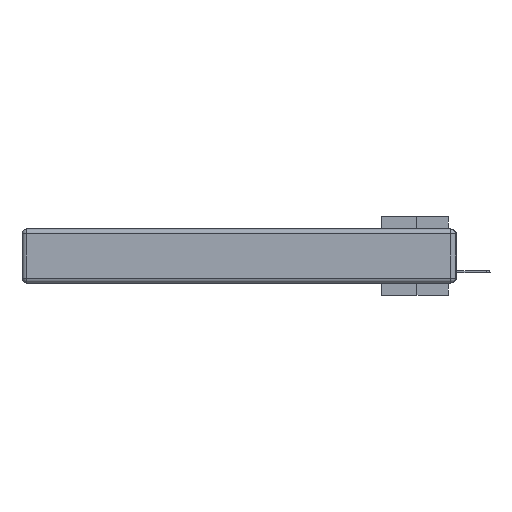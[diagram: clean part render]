
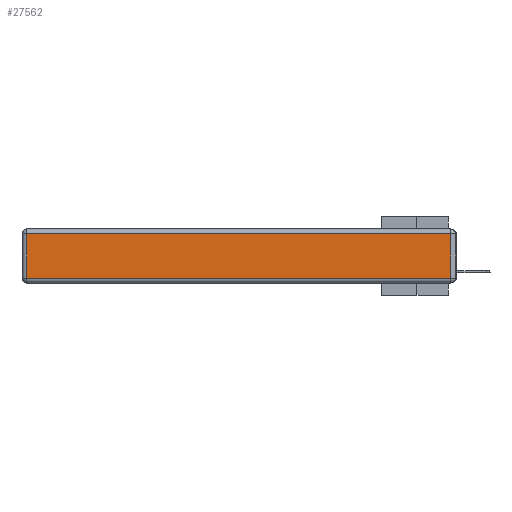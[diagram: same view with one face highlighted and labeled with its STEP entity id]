
A CAD part, left-side view. The second image highlights one B-rep face of the part: STEP entity #27562.
In plain terms, the highlighted planar face has unit normal (-1, 0, 0).
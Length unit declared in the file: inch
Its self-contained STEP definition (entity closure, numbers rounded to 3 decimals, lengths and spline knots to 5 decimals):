
#296 = EDGE_CURVE ( 'NONE', #33490, #36458, #23448, .T. ) ;
#3429 = DIRECTION ( 'NONE',  ( 0., -1., 0. ) ) ;
#3617 = AXIS2_PLACEMENT_3D ( 'NONE', #33273, #27860, #33509 ) ;
#4100 = LINE ( 'NONE', #26617, #32012 ) ;
#4236 = CARTESIAN_POINT ( 'NONE',  ( 0., 0.03, -0.03 ) ) ;
#4678 = EDGE_LOOP ( 'NONE', ( #19805, #11359, #30119, #31529 ) ) ;
#9135 = CARTESIAN_POINT ( 'NONE',  ( 0., 2.72, -0.313 ) ) ;
#11359 = ORIENTED_EDGE ( 'NONE', *, *, #21497, .T. ) ;
#11475 = DIRECTION ( 'NONE',  ( 0., 1., 0. ) ) ;
#11757 = EDGE_CURVE ( 'NONE', #20906, #33490, #23233, .T. ) ;
#13378 = FACE_OUTER_BOUND ( 'NONE', #4678, .T. ) ;
#16796 = CARTESIAN_POINT ( 'NONE',  ( 0., 0.03, -0.343 ) ) ;
#18258 = VECTOR ( 'NONE', #11475, 39.37008 ) ;
#18913 = VERTEX_POINT ( 'NONE', #28875 ) ;
#19805 = ORIENTED_EDGE ( 'NONE', *, *, #25335, .T. ) ;
#20906 = VERTEX_POINT ( 'NONE', #4236 ) ;
#21497 = EDGE_CURVE ( 'NONE', #18913, #20906, #30073, .T. ) ;
#22880 = CARTESIAN_POINT ( 'NONE',  ( 0., 2.72, -0.03 ) ) ;
#23233 = LINE ( 'NONE', #36907, #18258 ) ;
#23448 = LINE ( 'NONE', #36123, #31992 ) ;
#24617 = PLANE ( 'NONE',  #3617 ) ;
#25335 = EDGE_CURVE ( 'NONE', #36458, #18913, #4100, .T. ) ;
#26617 = CARTESIAN_POINT ( 'NONE',  ( 0., 0., -0.313 ) ) ;
#27562 = ADVANCED_FACE ( 'NONE', ( #13378 ), #24617, .T. ) ;
#27860 = DIRECTION ( 'NONE',  ( -1., 0., 0. ) ) ;
#28875 = CARTESIAN_POINT ( 'NONE',  ( 0., 0.03, -0.313 ) ) ;
#30073 = LINE ( 'NONE', #16796, #30951 ) ;
#30119 = ORIENTED_EDGE ( 'NONE', *, *, #11757, .T. ) ;
#30366 = DIRECTION ( 'NONE',  ( 0., 0., -1. ) ) ;
#30951 = VECTOR ( 'NONE', #31429, 39.37008 ) ;
#31429 = DIRECTION ( 'NONE',  ( 0., 0., 1. ) ) ;
#31529 = ORIENTED_EDGE ( 'NONE', *, *, #296, .T. ) ;
#31992 = VECTOR ( 'NONE', #30366, 39.37008 ) ;
#32012 = VECTOR ( 'NONE', #3429, 39.37008 ) ;
#33273 = CARTESIAN_POINT ( 'NONE',  ( 0., 0., -0.343 ) ) ;
#33490 = VERTEX_POINT ( 'NONE', #22880 ) ;
#33509 = DIRECTION ( 'NONE',  ( 0., 0., 1. ) ) ;
#36123 = CARTESIAN_POINT ( 'NONE',  ( 0., 2.72, -0.343 ) ) ;
#36458 = VERTEX_POINT ( 'NONE', #9135 ) ;
#36907 = CARTESIAN_POINT ( 'NONE',  ( 0., 2.75, -0.03 ) ) ;
